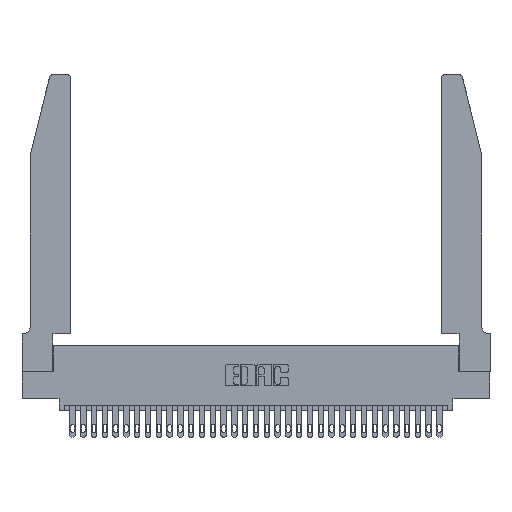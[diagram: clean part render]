
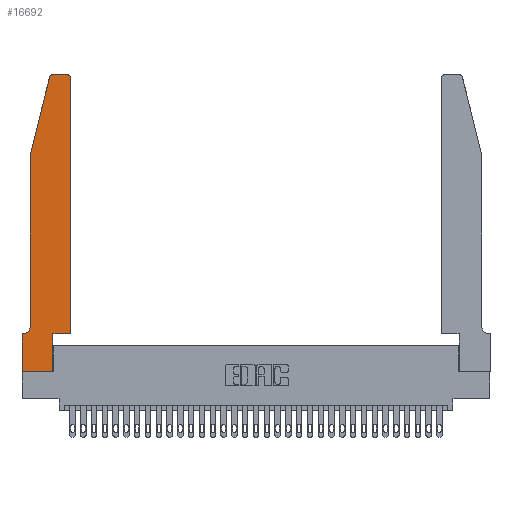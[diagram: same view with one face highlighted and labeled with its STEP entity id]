
A CAD part, top view. The second image highlights one B-rep face of the part: STEP entity #16692.
In plain terms, the highlighted planar face has unit normal (0, 0, 1).
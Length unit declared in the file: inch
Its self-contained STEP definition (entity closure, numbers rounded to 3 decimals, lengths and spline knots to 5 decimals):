
#153 = VERTEX_POINT ( 'NONE', #5317 ) ;
#290 = VERTEX_POINT ( 'NONE', #18812 ) ;
#518 = EDGE_CURVE ( 'NONE', #8809, #153, #32143, .T. ) ;
#889 = CARTESIAN_POINT ( 'NONE',  ( 0.2865, 0., 0.37 ) ) ;
#1686 = CARTESIAN_POINT ( 'NONE',  ( 0., 0., 0.37 ) ) ;
#1910 = ORIENTED_EDGE ( 'NONE', *, *, #30208, .T. ) ;
#1930 = LINE ( 'NONE', #31072, #2735 ) ;
#2300 = DIRECTION ( 'NONE',  ( 1., 0., 0. ) ) ;
#2543 = DIRECTION ( 'NONE',  ( 0., -1., 0. ) ) ;
#2735 = VECTOR ( 'NONE', #2543, 39.37008 ) ;
#3337 = CARTESIAN_POINT ( 'NONE',  ( 0.0755, 2., 0.37 ) ) ;
#3642 = EDGE_CURVE ( 'NONE', #290, #15681, #28428, .T. ) ;
#5108 = DIRECTION ( 'NONE',  ( 0., 1., 0. ) ) ;
#5317 = CARTESIAN_POINT ( 'NONE',  ( 0.0055, 0.35, 0.37 ) ) ;
#5348 = LINE ( 'NONE', #26098, #6524 ) ;
#5606 = AXIS2_PLACEMENT_3D ( 'NONE', #6405, #14035, #31988 ) ;
#5846 = DIRECTION ( 'NONE',  ( 0., 0., 1. ) ) ;
#6285 = ORIENTED_EDGE ( 'NONE', *, *, #14132, .T. ) ;
#6299 = ORIENTED_EDGE ( 'NONE', *, *, #32482, .T. ) ;
#6405 = CARTESIAN_POINT ( 'NONE',  ( 0.4205, 2.72, 0.37 ) ) ;
#6524 = VECTOR ( 'NONE', #10857, 39.37008 ) ;
#7216 = VECTOR ( 'NONE', #5108, 39.37008 ) ;
#8192 = DIRECTION ( 'NONE',  ( 1., 0., 0. ) ) ;
#8591 = EDGE_CURVE ( 'NONE', #21049, #29067, #14034, .T. ) ;
#8630 = ORIENTED_EDGE ( 'NONE', *, *, #27760, .T. ) ;
#8809 = VERTEX_POINT ( 'NONE', #21048 ) ;
#8839 = EDGE_CURVE ( 'NONE', #21810, #17316, #5348, .T. ) ;
#8892 = EDGE_CURVE ( 'NONE', #25343, #29394, #27277, .T. ) ;
#9326 = VECTOR ( 'NONE', #27562, 39.37008 ) ;
#10070 = CARTESIAN_POINT ( 'NONE',  ( 0., 0., 0.37 ) ) ;
#10857 = DIRECTION ( 'NONE',  ( -0.239, -0.971, 0. ) ) ;
#10908 = LINE ( 'NONE', #28752, #30578 ) ;
#12292 = FACE_OUTER_BOUND ( 'NONE', #30733, .T. ) ;
#12880 = CARTESIAN_POINT ( 'NONE',  ( 0.0055, 0.42, 0.37 ) ) ;
#13064 = VECTOR ( 'NONE', #31365, 39.37008 ) ;
#13694 = CARTESIAN_POINT ( 'NONE',  ( 0.284, 2.72, 0.37 ) ) ;
#14034 = LINE ( 'NONE', #30505, #7216 ) ;
#14035 = DIRECTION ( 'NONE',  ( 0., 0., 1. ) ) ;
#14132 = EDGE_CURVE ( 'NONE', #29394, #22030, #23775, .T. ) ;
#14311 = AXIS2_PLACEMENT_3D ( 'NONE', #12880, #17833, #17728 ) ;
#15114 = EDGE_CURVE ( 'NONE', #153, #26496, #10908, .T. ) ;
#15681 = VERTEX_POINT ( 'NONE', #16539 ) ;
#15838 = DIRECTION ( 'NONE',  ( -1., 0., 0. ) ) ;
#15922 = DIRECTION ( 'NONE',  ( 0., 0., 1. ) ) ;
#16539 = CARTESIAN_POINT ( 'NONE',  ( 0.284, 2.75, 0.37 ) ) ;
#16692 = ADVANCED_FACE ( 'NONE', ( #12292 ), #23416, .T. ) ;
#17155 = CARTESIAN_POINT ( 'NONE',  ( 0.2605, 2.75, 0.37 ) ) ;
#17316 = VERTEX_POINT ( 'NONE', #3337 ) ;
#17473 = DIRECTION ( 'NONE',  ( -1., 0., 0. ) ) ;
#17728 = DIRECTION ( 'NONE',  ( -1., 0., 0. ) ) ;
#17833 = DIRECTION ( 'NONE',  ( 0., 0., -1. ) ) ;
#18355 = CARTESIAN_POINT ( 'NONE',  ( 0.4505, 0.35, 0.37 ) ) ;
#18368 = CARTESIAN_POINT ( 'NONE',  ( 0., 0., 0.37 ) ) ;
#18440 = VECTOR ( 'NONE', #30938, 39.37008 ) ;
#18638 = ORIENTED_EDGE ( 'NONE', *, *, #3642, .T. ) ;
#18812 = CARTESIAN_POINT ( 'NONE',  ( 0.4205, 2.75, 0.37 ) ) ;
#19230 = ORIENTED_EDGE ( 'NONE', *, *, #29378, .T. ) ;
#20841 = CARTESIAN_POINT ( 'NONE',  ( 0.25487, 2.72718, 0.37 ) ) ;
#20954 = LINE ( 'NONE', #1686, #23761 ) ;
#20959 = CARTESIAN_POINT ( 'NONE',  ( 0., 0.35, 0.37 ) ) ;
#21048 = CARTESIAN_POINT ( 'NONE',  ( 0.0755, 0.42, 0.37 ) ) ;
#21049 = VERTEX_POINT ( 'NONE', #32417 ) ;
#21070 = ORIENTED_EDGE ( 'NONE', *, *, #15114, .T. ) ;
#21810 = VERTEX_POINT ( 'NONE', #20841 ) ;
#21964 = AXIS2_PLACEMENT_3D ( 'NONE', #13694, #5846, #8192 ) ;
#22030 = VERTEX_POINT ( 'NONE', #26783 ) ;
#23416 = PLANE ( 'NONE',  #33125 ) ;
#23761 = VECTOR ( 'NONE', #30557, 39.37008 ) ;
#23775 = LINE ( 'NONE', #24955, #9326 ) ;
#23950 = CIRCLE ( 'NONE', #5606, 0.03 ) ;
#24234 = ORIENTED_EDGE ( 'NONE', *, *, #518, .T. ) ;
#24340 = CARTESIAN_POINT ( 'NONE',  ( 0., 0.35, 0.37 ) ) ;
#24955 = CARTESIAN_POINT ( 'NONE',  ( 0.2865, 0.35, 0.37 ) ) ;
#25343 = VERTEX_POINT ( 'NONE', #10070 ) ;
#25602 = EDGE_CURVE ( 'NONE', #22030, #21049, #31105, .T. ) ;
#26098 = CARTESIAN_POINT ( 'NONE',  ( 0.0755, 2., 0.37 ) ) ;
#26496 = VERTEX_POINT ( 'NONE', #24340 ) ;
#26783 = CARTESIAN_POINT ( 'NONE',  ( 0.2865, 0.35, 0.37 ) ) ;
#26895 = ORIENTED_EDGE ( 'NONE', *, *, #8839, .T. ) ;
#27082 = ORIENTED_EDGE ( 'NONE', *, *, #8892, .T. ) ;
#27277 = LINE ( 'NONE', #18368, #18440 ) ;
#27462 = CIRCLE ( 'NONE', #21964, 0.03 ) ;
#27562 = DIRECTION ( 'NONE',  ( 0., 1., 0. ) ) ;
#27760 = EDGE_CURVE ( 'NONE', #29067, #290, #23950, .T. ) ;
#28428 = LINE ( 'NONE', #17155, #29608 ) ;
#28430 = ORIENTED_EDGE ( 'NONE', *, *, #8591, .T. ) ;
#28752 = CARTESIAN_POINT ( 'NONE',  ( 0.0755, 0.35, 0.37 ) ) ;
#29067 = VERTEX_POINT ( 'NONE', #32361 ) ;
#29378 = EDGE_CURVE ( 'NONE', #15681, #21810, #27462, .T. ) ;
#29394 = VERTEX_POINT ( 'NONE', #889 ) ;
#29608 = VECTOR ( 'NONE', #17473, 39.37008 ) ;
#29860 = ORIENTED_EDGE ( 'NONE', *, *, #25602, .T. ) ;
#30208 = EDGE_CURVE ( 'NONE', #26496, #25343, #20954, .T. ) ;
#30505 = CARTESIAN_POINT ( 'NONE',  ( 0.4505, 0.35, 0.37 ) ) ;
#30557 = DIRECTION ( 'NONE',  ( 0., -1., 0. ) ) ;
#30578 = VECTOR ( 'NONE', #15838, 39.37008 ) ;
#30733 = EDGE_LOOP ( 'NONE', ( #18638, #19230, #26895, #6299, #24234, #21070, #1910, #27082, #6285, #29860, #28430, #8630 ) ) ;
#30938 = DIRECTION ( 'NONE',  ( 1., 0., 0. ) ) ;
#31072 = CARTESIAN_POINT ( 'NONE',  ( 0.0755, 2., 0.37 ) ) ;
#31105 = LINE ( 'NONE', #18355, #13064 ) ;
#31365 = DIRECTION ( 'NONE',  ( 1., 0., 0. ) ) ;
#31988 = DIRECTION ( 'NONE',  ( 1., 0., 0. ) ) ;
#32143 = CIRCLE ( 'NONE', #14311, 0.07 ) ;
#32361 = CARTESIAN_POINT ( 'NONE',  ( 0.4505, 2.72, 0.37 ) ) ;
#32417 = CARTESIAN_POINT ( 'NONE',  ( 0.4505, 0.35, 0.37 ) ) ;
#32482 = EDGE_CURVE ( 'NONE', #17316, #8809, #1930, .T. ) ;
#33125 = AXIS2_PLACEMENT_3D ( 'NONE', #20959, #15922, #2300 ) ;
